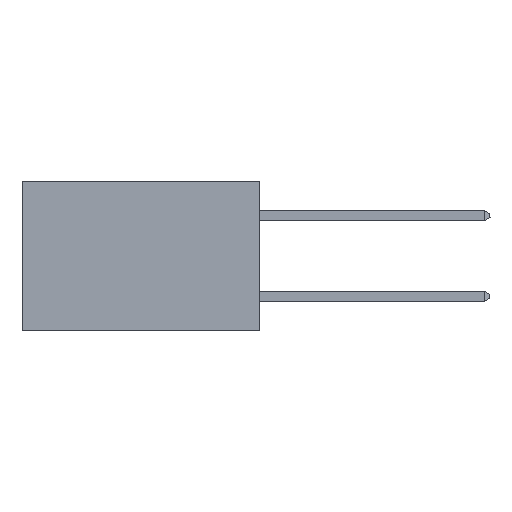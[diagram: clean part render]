
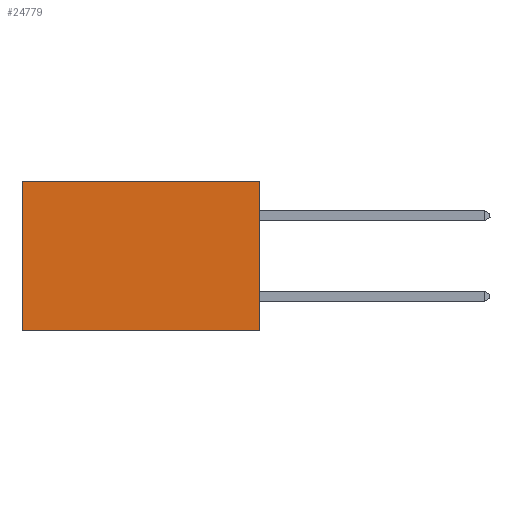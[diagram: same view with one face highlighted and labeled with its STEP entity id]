
A CAD part, left-side view. The second image highlights one B-rep face of the part: STEP entity #24779.
In plain terms, the highlighted planar face has unit normal (-1, 0, 0).
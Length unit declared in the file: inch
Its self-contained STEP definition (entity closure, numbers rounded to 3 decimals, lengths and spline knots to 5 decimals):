
#81 = AXIS2_PLACEMENT_3D ( 'NONE', #6756, #27452, #11940 ) ;
#688 = ORIENTED_EDGE ( 'NONE', *, *, #8086, .F. ) ;
#1109 = CARTESIAN_POINT ( 'NONE',  ( 0.277, 0., -0.37 ) ) ;
#3967 = DIRECTION ( 'NONE',  ( 0., 1., 0. ) ) ;
#4825 = LINE ( 'NONE', #19295, #30696 ) ;
#5502 = EDGE_CURVE ( 'NONE', #32825, #5836, #26996, .T. ) ;
#5836 = VERTEX_POINT ( 'NONE', #10065 ) ;
#6367 = VECTOR ( 'NONE', #26819, 39.37008 ) ;
#6756 = CARTESIAN_POINT ( 'NONE',  ( 0.277, 0., -0.37 ) ) ;
#8086 = EDGE_CURVE ( 'NONE', #32825, #26059, #10224, .T. ) ;
#10065 = CARTESIAN_POINT ( 'NONE',  ( 0.277, 0.59, 0. ) ) ;
#10224 = LINE ( 'NONE', #28830, #11838 ) ;
#10250 = EDGE_CURVE ( 'NONE', #26059, #24826, #4825, .T. ) ;
#11838 = VECTOR ( 'NONE', #15940, 39.37008 ) ;
#11870 = ORIENTED_EDGE ( 'NONE', *, *, #10250, .F. ) ;
#11940 = DIRECTION ( 'NONE',  ( 0., 0., -1. ) ) ;
#15658 = ORIENTED_EDGE ( 'NONE', *, *, #5502, .T. ) ;
#15940 = DIRECTION ( 'NONE',  ( 0., 0., -1. ) ) ;
#16241 = EDGE_CURVE ( 'NONE', #5836, #24826, #21933, .T. ) ;
#16721 = CARTESIAN_POINT ( 'NONE',  ( 0.277, 0., 0. ) ) ;
#17104 = CARTESIAN_POINT ( 'NONE',  ( 0.277, 0.59, -0.37 ) ) ;
#19295 = CARTESIAN_POINT ( 'NONE',  ( 0.277, 0., -0.37 ) ) ;
#19707 = DIRECTION ( 'NONE',  ( 0., 0., -1. ) ) ;
#19867 = CARTESIAN_POINT ( 'NONE',  ( 0.277, 0.59, -0.37 ) ) ;
#20343 = ORIENTED_EDGE ( 'NONE', *, *, #16241, .T. ) ;
#20917 = FACE_OUTER_BOUND ( 'NONE', #32162, .T. ) ;
#21125 = VECTOR ( 'NONE', #19707, 39.37008 ) ;
#21618 = CARTESIAN_POINT ( 'NONE',  ( 0.277, 0., 0. ) ) ;
#21933 = LINE ( 'NONE', #17104, #21125 ) ;
#24779 = ADVANCED_FACE ( 'NONE', ( #20917 ), #24810, .F. ) ;
#24810 = PLANE ( 'NONE',  #81 ) ;
#24826 = VERTEX_POINT ( 'NONE', #19867 ) ;
#26059 = VERTEX_POINT ( 'NONE', #1109 ) ;
#26819 = DIRECTION ( 'NONE',  ( 0., 1., 0. ) ) ;
#26996 = LINE ( 'NONE', #21618, #6367 ) ;
#27452 = DIRECTION ( 'NONE',  ( 1., 0., 0. ) ) ;
#28830 = CARTESIAN_POINT ( 'NONE',  ( 0.277, 0., -0.37 ) ) ;
#30696 = VECTOR ( 'NONE', #3967, 39.37008 ) ;
#32162 = EDGE_LOOP ( 'NONE', ( #20343, #11870, #688, #15658 ) ) ;
#32825 = VERTEX_POINT ( 'NONE', #16721 ) ;
